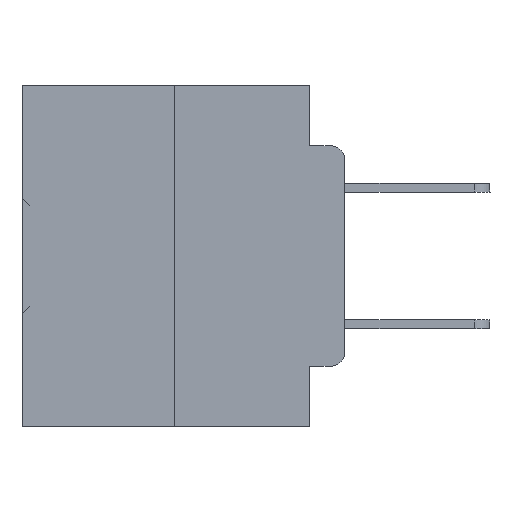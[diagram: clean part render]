
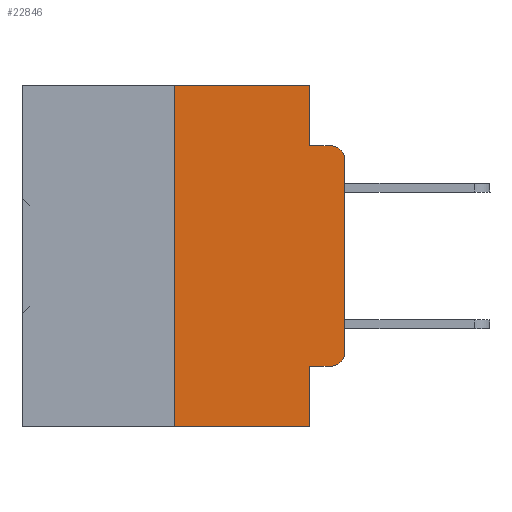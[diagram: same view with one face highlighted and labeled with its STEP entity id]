
A CAD part, left-side view. The second image highlights one B-rep face of the part: STEP entity #22846.
In plain terms, the highlighted planar face has unit normal (-1, 0, 0).
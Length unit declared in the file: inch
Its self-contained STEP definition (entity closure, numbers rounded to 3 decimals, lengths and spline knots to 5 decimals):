
#152 = CARTESIAN_POINT ( 'NONE',  ( 0., 0.051, 0. ) ) ;
#316 = LINE ( 'NONE', #19395, #15603 ) ;
#338 = EDGE_CURVE ( 'NONE', #19806, #25774, #316, .T. ) ;
#630 = CARTESIAN_POINT ( 'NONE',  ( 0., 0.25, 0. ) ) ;
#890 = CARTESIAN_POINT ( 'NONE',  ( 0., 0.051, -0.4115 ) ) ;
#1340 = ORIENTED_EDGE ( 'NONE', *, *, #11983, .T. ) ;
#2113 = VECTOR ( 'NONE', #19239, 39.37008 ) ;
#2175 = VERTEX_POINT ( 'NONE', #15352 ) ;
#3097 = VERTEX_POINT ( 'NONE', #10955 ) ;
#3224 = CARTESIAN_POINT ( 'NONE',  ( 0., 0., -0.3915 ) ) ;
#3265 = VERTEX_POINT ( 'NONE', #8691 ) ;
#3549 = DIRECTION ( 'NONE',  ( 0., -1., 0. ) ) ;
#3728 = AXIS2_PLACEMENT_3D ( 'NONE', #19517, #25993, #35713 ) ;
#4593 = VERTEX_POINT ( 'NONE', #3224 ) ;
#4636 = DIRECTION ( 'NONE',  ( 0., -1., 0. ) ) ;
#4984 = ORIENTED_EDGE ( 'NONE', *, *, #27439, .F. ) ;
#5181 = CARTESIAN_POINT ( 'NONE',  ( 0., 0.473, 0. ) ) ;
#6816 = CARTESIAN_POINT ( 'NONE',  ( 0., 0.02, -0.3915 ) ) ;
#7179 = VERTEX_POINT ( 'NONE', #38319 ) ;
#7827 = EDGE_CURVE ( 'NONE', #7179, #25774, #16090, .T. ) ;
#7829 = LINE ( 'NONE', #5181, #21049 ) ;
#7840 = CIRCLE ( 'NONE', #13010, 0.02 ) ;
#8370 = EDGE_CURVE ( 'NONE', #19806, #27243, #23154, .T. ) ;
#8691 = CARTESIAN_POINT ( 'NONE',  ( 0., 0., -0.1085 ) ) ;
#8961 = EDGE_CURVE ( 'NONE', #32683, #14431, #20244, .T. ) ;
#9350 = ORIENTED_EDGE ( 'NONE', *, *, #34095, .F. ) ;
#9498 = VECTOR ( 'NONE', #20489, 39.37008 ) ;
#9854 = DIRECTION ( 'NONE',  ( 0., -1., 0. ) ) ;
#10955 = CARTESIAN_POINT ( 'NONE',  ( 0., 0.02, -0.4115 ) ) ;
#11983 = EDGE_CURVE ( 'NONE', #3265, #14431, #21217, .T. ) ;
#12122 = CARTESIAN_POINT ( 'NONE',  ( 0., 0.25, 0. ) ) ;
#13010 = AXIS2_PLACEMENT_3D ( 'NONE', #6816, #13285, #28891 ) ;
#13285 = DIRECTION ( 'NONE',  ( -1., 0., 0. ) ) ;
#13420 = DIRECTION ( 'NONE',  ( 0., 0., 1. ) ) ;
#13528 = FACE_OUTER_BOUND ( 'NONE', #21620, .T. ) ;
#14431 = VERTEX_POINT ( 'NONE', #18176 ) ;
#14582 = EDGE_CURVE ( 'NONE', #3097, #4593, #7840, .T. ) ;
#15243 = VECTOR ( 'NONE', #13420, 39.37008 ) ;
#15305 = CARTESIAN_POINT ( 'NONE',  ( 0., 0.25, -0.5 ) ) ;
#15352 = CARTESIAN_POINT ( 'NONE',  ( 0., 0.051, 0. ) ) ;
#15603 = VECTOR ( 'NONE', #9854, 39.37008 ) ;
#15690 = ORIENTED_EDGE ( 'NONE', *, *, #7827, .F. ) ;
#15962 = CARTESIAN_POINT ( 'NONE',  ( 0., 0.473, 0. ) ) ;
#16090 = LINE ( 'NONE', #24072, #27499 ) ;
#17639 = VECTOR ( 'NONE', #3549, 39.37008 ) ;
#18087 = ORIENTED_EDGE ( 'NONE', *, *, #39127, .T. ) ;
#18176 = CARTESIAN_POINT ( 'NONE',  ( 0., 0.02, -0.0885 ) ) ;
#19239 = DIRECTION ( 'NONE',  ( 0., 0., -1. ) ) ;
#19395 = CARTESIAN_POINT ( 'NONE',  ( 0., 0.473, -0.5 ) ) ;
#19517 = CARTESIAN_POINT ( 'NONE',  ( 0., 0.02, -0.1085 ) ) ;
#19806 = VERTEX_POINT ( 'NONE', #15305 ) ;
#20244 = LINE ( 'NONE', #33000, #35572 ) ;
#20489 = DIRECTION ( 'NONE',  ( 0., 0., 1. ) ) ;
#20544 = ORIENTED_EDGE ( 'NONE', *, *, #8370, .F. ) ;
#20796 = ORIENTED_EDGE ( 'NONE', *, *, #14582, .T. ) ;
#21049 = VECTOR ( 'NONE', #32953, 39.37008 ) ;
#21217 = CIRCLE ( 'NONE', #3728, 0.02 ) ;
#21620 = EDGE_LOOP ( 'NONE', ( #18087, #1340, #34948, #9350, #4984, #20544, #28223, #15690, #24178, #20796 ) ) ;
#21986 = DIRECTION ( 'NONE',  ( 0., 0., -1. ) ) ;
#22195 = LINE ( 'NONE', #890, #17639 ) ;
#22846 = ADVANCED_FACE ( 'NONE', ( #13528 ), #25888, .F. ) ;
#23154 = LINE ( 'NONE', #630, #15243 ) ;
#23290 = EDGE_CURVE ( 'NONE', #7179, #3097, #22195, .T. ) ;
#23443 = DIRECTION ( 'NONE',  ( 1., 0., 0. ) ) ;
#24072 = CARTESIAN_POINT ( 'NONE',  ( 0., 0.051, 0. ) ) ;
#24178 = ORIENTED_EDGE ( 'NONE', *, *, #23290, .T. ) ;
#25774 = VERTEX_POINT ( 'NONE', #36377 ) ;
#25888 = PLANE ( 'NONE',  #39637 ) ;
#25993 = DIRECTION ( 'NONE',  ( -1., 0., 0. ) ) ;
#26551 = CARTESIAN_POINT ( 'NONE',  ( 0., 0., 0. ) ) ;
#27243 = VERTEX_POINT ( 'NONE', #12122 ) ;
#27439 = EDGE_CURVE ( 'NONE', #27243, #2175, #7829, .T. ) ;
#27499 = VECTOR ( 'NONE', #21986, 39.37008 ) ;
#28223 = ORIENTED_EDGE ( 'NONE', *, *, #338, .T. ) ;
#28891 = DIRECTION ( 'NONE',  ( 0., 0., -1. ) ) ;
#29710 = DIRECTION ( 'NONE',  ( 0., 0., -1. ) ) ;
#32442 = LINE ( 'NONE', #26551, #9498 ) ;
#32683 = VERTEX_POINT ( 'NONE', #36254 ) ;
#32953 = DIRECTION ( 'NONE',  ( 0., -1., 0. ) ) ;
#33000 = CARTESIAN_POINT ( 'NONE',  ( 0., 0.051, -0.0885 ) ) ;
#34095 = EDGE_CURVE ( 'NONE', #2175, #32683, #37663, .T. ) ;
#34948 = ORIENTED_EDGE ( 'NONE', *, *, #8961, .F. ) ;
#35572 = VECTOR ( 'NONE', #4636, 39.37008 ) ;
#35713 = DIRECTION ( 'NONE',  ( 0., 0., -1. ) ) ;
#36254 = CARTESIAN_POINT ( 'NONE',  ( 0., 0.051, -0.0885 ) ) ;
#36377 = CARTESIAN_POINT ( 'NONE',  ( 0., 0.051, -0.5 ) ) ;
#37663 = LINE ( 'NONE', #152, #2113 ) ;
#38319 = CARTESIAN_POINT ( 'NONE',  ( 0., 0.051, -0.4115 ) ) ;
#39127 = EDGE_CURVE ( 'NONE', #4593, #3265, #32442, .T. ) ;
#39637 = AXIS2_PLACEMENT_3D ( 'NONE', #15962, #23443, #29710 ) ;
